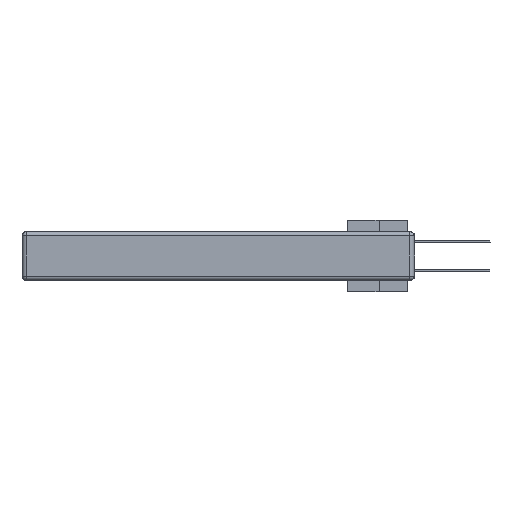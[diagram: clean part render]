
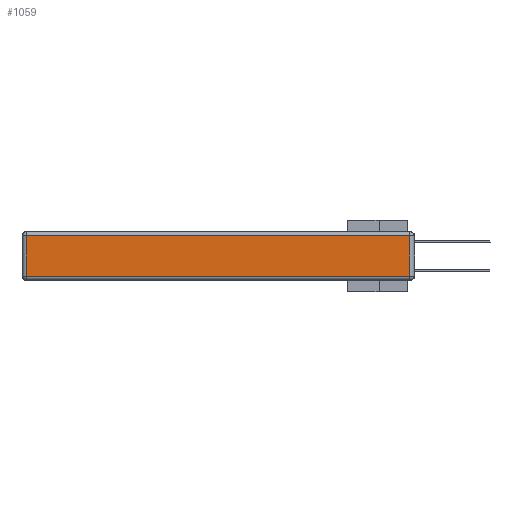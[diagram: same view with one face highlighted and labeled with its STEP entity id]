
A CAD part, left-side view. The second image highlights one B-rep face of the part: STEP entity #1059.
In plain terms, the highlighted planar face has unit normal (-1, 0, 0).
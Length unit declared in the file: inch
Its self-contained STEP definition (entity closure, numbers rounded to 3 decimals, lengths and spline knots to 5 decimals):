
#1059 = ADVANCED_FACE ( 'NONE', ( #18601 ), #13612, .T. ) ;
#1070 = EDGE_CURVE ( 'NONE', #18090, #38982, #28561, .T. ) ;
#5183 = EDGE_CURVE ( 'NONE', #38982, #7664, #22033, .T. ) ;
#7664 = VERTEX_POINT ( 'NONE', #25567 ) ;
#8770 = VECTOR ( 'NONE', #28107, 39.37008 ) ;
#12049 = CARTESIAN_POINT ( 'NONE',  ( 0., 0.03, -0.03 ) ) ;
#12225 = VERTEX_POINT ( 'NONE', #32745 ) ;
#13612 = PLANE ( 'NONE',  #16012 ) ;
#15944 = EDGE_CURVE ( 'NONE', #12225, #18090, #21800, .T. ) ;
#16012 = AXIS2_PLACEMENT_3D ( 'NONE', #34811, #22519, #16555 ) ;
#16555 = DIRECTION ( 'NONE',  ( 0., 0., 1. ) ) ;
#18090 = VERTEX_POINT ( 'NONE', #12049 ) ;
#18601 = FACE_OUTER_BOUND ( 'NONE', #27339, .T. ) ;
#19434 = VECTOR ( 'NONE', #25606, 39.37008 ) ;
#19797 = CARTESIAN_POINT ( 'NONE',  ( 0., 0., -0.313 ) ) ;
#20072 = DIRECTION ( 'NONE',  ( 0., -1., 0. ) ) ;
#20928 = LINE ( 'NONE', #19797, #29899 ) ;
#21276 = EDGE_CURVE ( 'NONE', #7664, #12225, #20928, .T. ) ;
#21800 = LINE ( 'NONE', #31697, #19434 ) ;
#21906 = VECTOR ( 'NONE', #26076, 39.37008 ) ;
#22033 = LINE ( 'NONE', #30602, #8770 ) ;
#22519 = DIRECTION ( 'NONE',  ( -1., 0., 0. ) ) ;
#22668 = ORIENTED_EDGE ( 'NONE', *, *, #5183, .T. ) ;
#25239 = CARTESIAN_POINT ( 'NONE',  ( 0., 2.72, -0.03 ) ) ;
#25567 = CARTESIAN_POINT ( 'NONE',  ( 0., 2.72, -0.313 ) ) ;
#25606 = DIRECTION ( 'NONE',  ( 0., 0., 1. ) ) ;
#26076 = DIRECTION ( 'NONE',  ( 0., 1., 0. ) ) ;
#27339 = EDGE_LOOP ( 'NONE', ( #28506, #33132, #34007, #22668 ) ) ;
#28107 = DIRECTION ( 'NONE',  ( 0., 0., -1. ) ) ;
#28337 = CARTESIAN_POINT ( 'NONE',  ( 0., 2.75, -0.03 ) ) ;
#28506 = ORIENTED_EDGE ( 'NONE', *, *, #21276, .T. ) ;
#28561 = LINE ( 'NONE', #28337, #21906 ) ;
#29899 = VECTOR ( 'NONE', #20072, 39.37008 ) ;
#30602 = CARTESIAN_POINT ( 'NONE',  ( 0., 2.72, -0.343 ) ) ;
#31697 = CARTESIAN_POINT ( 'NONE',  ( 0., 0.03, -0.343 ) ) ;
#32745 = CARTESIAN_POINT ( 'NONE',  ( 0., 0.03, -0.313 ) ) ;
#33132 = ORIENTED_EDGE ( 'NONE', *, *, #15944, .T. ) ;
#34007 = ORIENTED_EDGE ( 'NONE', *, *, #1070, .T. ) ;
#34811 = CARTESIAN_POINT ( 'NONE',  ( 0., 0., -0.343 ) ) ;
#38982 = VERTEX_POINT ( 'NONE', #25239 ) ;
